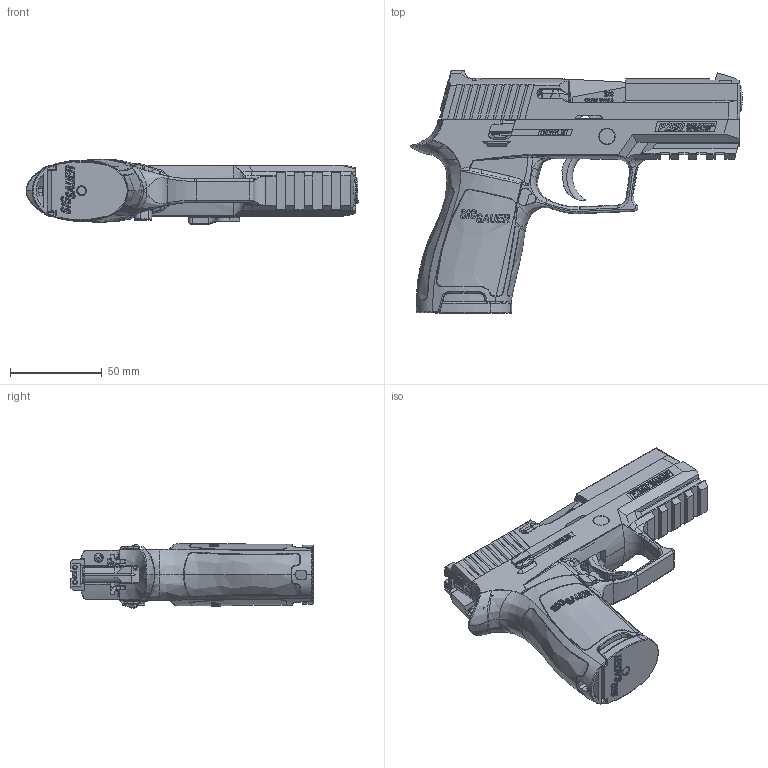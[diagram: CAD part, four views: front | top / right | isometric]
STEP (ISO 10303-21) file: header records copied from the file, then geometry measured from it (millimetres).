
FILE_DESCRIPTION(/* description */ (''),/* implementation_level */ '2;1');
FILE_NAME(/* name */ 'Final Build.stp',/* time_stamp */ '2014-07-30T14:17:52-04:00',/* author */ ('Dave'),/* organization */ (''),/* preprocessor_version */ 'ST-DEVELOPER v15.6',/* originating_system */ 'Autodesk Inventor 2015',/* authorisation */ '');
FILE_SCHEMA (('AUTOMOTIVE_DESIGN { 1 0 10303 214 3 1 1 }'));
Products named in the file (37): Slide_1; Barrel; Extractor Spring; Extractor; Firing Pin Spring; Firing Pin; Frame; Front Extractor Spring Guide; Front Sight; Hammer Strut Pin; Hammer; Large Mainspring; Magazine Catch Stop; Magazine Catch; Magazine Floorplate; Magazine Insert; Magazine Release Spring; Rear Extractor Spring Guide; Rear Sight; Recoil Spring Guide; Recoil Spring; Safety Lever; Safety Lock; Safety Locking Spring; Slide Catch Lever Pin; Slide Catch Lever; Small Mainspring; Spring Pin; Takedown Lever O-Ring; Takedown Lever; Trigger Bar; Trigger; Polymer v5 latest backup; Hammer Pivot Pin; Magazine Tube - Copy; Part31; Final Build
Bounding box: 181.43 x 132.31 x 35.8 mm (x, y, z)
Volume: 161824 mm3; surface area: 141333.6 mm2
Topology: 36 solids, 36 shells, 4729 faces, 12875 edges, 8367 vertices
Faces by surface type: plane 2489, bspline 1451, cylinder 672, torus 82, cone 23, sphere 12
Full cylindrical faces by diameter (mm): 1.511 x1, 1.651 x1, 1.753 x1, 1.778 x1, 2.159 x1, 2.172 x1, 2.257 x1, 2.375 x1, 2.426 x1, 2.477 x1, 2.527 x2, 2.616 x1, 2.671 x2, 2.756 x1, 2.769 x1, 2.896 x1, 2.921 x2, 2.959 x1, 3.048 x2, 3.061 x3, 3.086 x1, 3.302 x1, 3.757 x2, 3.873 x1, 3.912 x1, 3.962 x1, 3.988 x1, 4.039 x1, 4.089 x2, 4.432 x1
Entity records: 196880 total; most frequent: CARTESIAN_POINT 86538, ORIENTED_EDGE 25364, DIRECTION 18084, EDGE_CURVE 12682, VERTEX_POINT 8323, LINE 7496, VECTOR 7496, AXIS2_PLACEMENT_3D 5294
